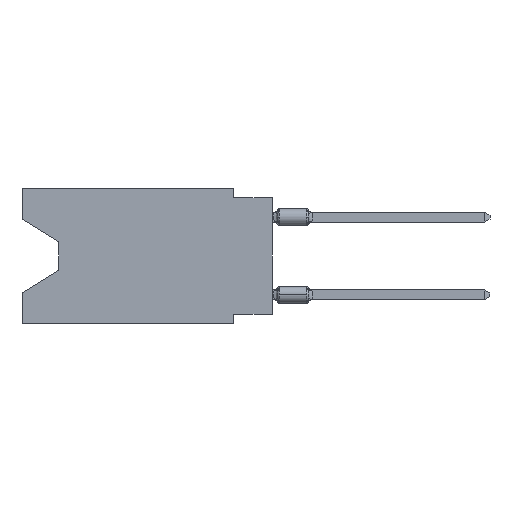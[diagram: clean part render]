
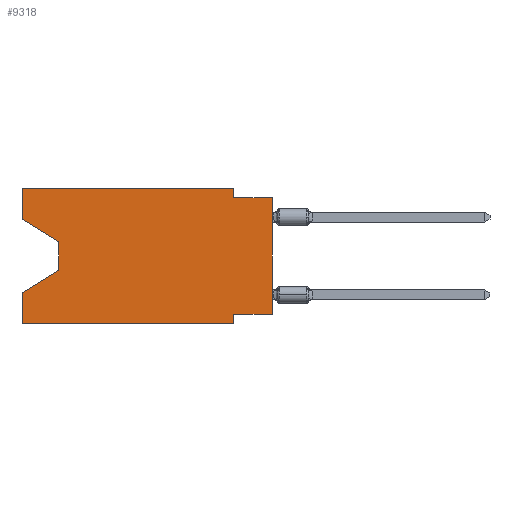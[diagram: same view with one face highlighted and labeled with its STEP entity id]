
A CAD part, left-side view. The second image highlights one B-rep face of the part: STEP entity #9318.
In plain terms, the highlighted planar face has unit normal (-1, 0, 0).
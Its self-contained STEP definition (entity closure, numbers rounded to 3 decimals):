
#119 = DIRECTION ( 'NONE',  ( 0., -0.855, -0.519 ) ) ;
#286 = CARTESIAN_POINT ( 'NONE',  ( 0., 16.383, 0. ) ) ;
#293 = VECTOR ( 'NONE', #8995, 1000. ) ;
#487 = EDGE_LOOP ( 'NONE', ( #8779, #12676, #13603, #1640, #14141, #2766, #3883, #6913, #11118, #13577, #760, #15820 ) ) ;
#689 = EDGE_CURVE ( 'NONE', #14110, #15507, #8025, .T. ) ;
#760 = ORIENTED_EDGE ( 'NONE', *, *, #9968, .F. ) ;
#988 = CARTESIAN_POINT ( 'NONE',  ( 0., 2.54, -8.89 ) ) ;
#1004 = VERTEX_POINT ( 'NONE', #4857 ) ;
#1427 = DIRECTION ( 'NONE',  ( 0., 0., -1. ) ) ;
#1616 = CARTESIAN_POINT ( 'NONE',  ( 0., 16.383, -8.89 ) ) ;
#1617 = AXIS2_PLACEMENT_3D ( 'NONE', #15998, #2168, #8337 ) ;
#1640 = ORIENTED_EDGE ( 'NONE', *, *, #5304, .F. ) ;
#1665 = LINE ( 'NONE', #4486, #16188 ) ;
#1762 = CARTESIAN_POINT ( 'NONE',  ( 0., 13.97, -5.385 ) ) ;
#1956 = VECTOR ( 'NONE', #12946, 1000. ) ;
#2101 = VECTOR ( 'NONE', #9533, 1000. ) ;
#2168 = DIRECTION ( 'NONE',  ( 1., 0., 0. ) ) ;
#2461 = VERTEX_POINT ( 'NONE', #4972 ) ;
#2766 = ORIENTED_EDGE ( 'NONE', *, *, #3567, .F. ) ;
#2842 = CARTESIAN_POINT ( 'NONE',  ( 0., 16.383, 0. ) ) ;
#2948 = CARTESIAN_POINT ( 'NONE',  ( 0., 0., -0.635 ) ) ;
#3024 = EDGE_CURVE ( 'NONE', #15430, #4402, #8748, .T. ) ;
#3173 = EDGE_CURVE ( 'NONE', #15507, #14469, #10854, .T. ) ;
#3236 = CARTESIAN_POINT ( 'NONE',  ( 0., 2.54, 0. ) ) ;
#3567 = EDGE_CURVE ( 'NONE', #1004, #7500, #13640, .T. ) ;
#3883 = ORIENTED_EDGE ( 'NONE', *, *, #8010, .F. ) ;
#3884 = LINE ( 'NONE', #1616, #17358 ) ;
#3995 = EDGE_CURVE ( 'NONE', #13683, #7500, #3884, .T. ) ;
#4402 = VERTEX_POINT ( 'NONE', #15620 ) ;
#4486 = CARTESIAN_POINT ( 'NONE',  ( 0., 0., -8.255 ) ) ;
#4857 = CARTESIAN_POINT ( 'NONE',  ( 0., 2.54, -8.255 ) ) ;
#4900 = CARTESIAN_POINT ( 'NONE',  ( 0., 16.383, -6.852 ) ) ;
#4905 = DIRECTION ( 'NONE',  ( 0., 0.855, -0.519 ) ) ;
#4957 = EDGE_CURVE ( 'NONE', #2461, #18977, #6547, .T. ) ;
#4972 = CARTESIAN_POINT ( 'NONE',  ( 0., 16.383, -2.038 ) ) ;
#5265 = CARTESIAN_POINT ( 'NONE',  ( 0., 13.97, -3.505 ) ) ;
#5304 = EDGE_CURVE ( 'NONE', #13683, #14469, #6423, .T. ) ;
#5669 = CARTESIAN_POINT ( 'NONE',  ( 0., 16.383, -8.89 ) ) ;
#5997 = DIRECTION ( 'NONE',  ( 0., 0., -1. ) ) ;
#6281 = CARTESIAN_POINT ( 'NONE',  ( 0., 2.54, -8.89 ) ) ;
#6423 = LINE ( 'NONE', #11070, #12446 ) ;
#6497 = CARTESIAN_POINT ( 'NONE',  ( 0., 13.97, -3.505 ) ) ;
#6547 = LINE ( 'NONE', #286, #9567 ) ;
#6851 = CARTESIAN_POINT ( 'NONE',  ( 0., 13.97, -5.385 ) ) ;
#6913 = ORIENTED_EDGE ( 'NONE', *, *, #9634, .T. ) ;
#7500 = VERTEX_POINT ( 'NONE', #988 ) ;
#7670 = VECTOR ( 'NONE', #4905, 1000. ) ;
#8010 = EDGE_CURVE ( 'NONE', #14268, #1004, #1665, .T. ) ;
#8025 = LINE ( 'NONE', #6497, #2101 ) ;
#8315 = LINE ( 'NONE', #9526, #1956 ) ;
#8337 = DIRECTION ( 'NONE',  ( 0., 0., -1. ) ) ;
#8748 = LINE ( 'NONE', #13669, #19560 ) ;
#8779 = ORIENTED_EDGE ( 'NONE', *, *, #19073, .T. ) ;
#8995 = DIRECTION ( 'NONE',  ( 0., -1., 0. ) ) ;
#9318 = ADVANCED_FACE ( 'NONE', ( #11354 ), #9847, .F. ) ;
#9526 = CARTESIAN_POINT ( 'NONE',  ( 0., 0., 0. ) ) ;
#9533 = DIRECTION ( 'NONE',  ( 0., 0., -1. ) ) ;
#9567 = VECTOR ( 'NONE', #14119, 1000. ) ;
#9634 = EDGE_CURVE ( 'NONE', #14268, #19158, #8315, .T. ) ;
#9847 = PLANE ( 'NONE',  #1617 ) ;
#9968 = EDGE_CURVE ( 'NONE', #18977, #15430, #15447, .T. ) ;
#10450 = DIRECTION ( 'NONE',  ( 0., 1., 0. ) ) ;
#10854 = LINE ( 'NONE', #1762, #7670 ) ;
#10906 = DIRECTION ( 'NONE',  ( 0., -1., 0. ) ) ;
#11070 = CARTESIAN_POINT ( 'NONE',  ( 0., 16.383, 0. ) ) ;
#11118 = ORIENTED_EDGE ( 'NONE', *, *, #13830, .F. ) ;
#11354 = FACE_OUTER_BOUND ( 'NONE', #487, .T. ) ;
#12030 = CARTESIAN_POINT ( 'NONE',  ( 0., 16.383, -2.038 ) ) ;
#12446 = VECTOR ( 'NONE', #12779, 1000. ) ;
#12676 = ORIENTED_EDGE ( 'NONE', *, *, #689, .T. ) ;
#12779 = DIRECTION ( 'NONE',  ( 0., 0., 1. ) ) ;
#12826 = VECTOR ( 'NONE', #1427, 1000. ) ;
#12894 = VECTOR ( 'NONE', #119, 1000. ) ;
#12946 = DIRECTION ( 'NONE',  ( 0., 0., 1. ) ) ;
#13450 = CARTESIAN_POINT ( 'NONE',  ( 0., 16.383, 0. ) ) ;
#13577 = ORIENTED_EDGE ( 'NONE', *, *, #3024, .F. ) ;
#13603 = ORIENTED_EDGE ( 'NONE', *, *, #3173, .T. ) ;
#13640 = LINE ( 'NONE', #6281, #12826 ) ;
#13669 = CARTESIAN_POINT ( 'NONE',  ( 0., 2.54, 0. ) ) ;
#13683 = VERTEX_POINT ( 'NONE', #5669 ) ;
#13830 = EDGE_CURVE ( 'NONE', #4402, #19158, #16777, .T. ) ;
#13957 = LINE ( 'NONE', #12030, #12894 ) ;
#14110 = VERTEX_POINT ( 'NONE', #5265 ) ;
#14119 = DIRECTION ( 'NONE',  ( 0., 0., 1. ) ) ;
#14141 = ORIENTED_EDGE ( 'NONE', *, *, #3995, .T. ) ;
#14268 = VERTEX_POINT ( 'NONE', #16206 ) ;
#14469 = VERTEX_POINT ( 'NONE', #4900 ) ;
#15246 = DIRECTION ( 'NONE',  ( 0., -1., 0. ) ) ;
#15430 = VERTEX_POINT ( 'NONE', #3236 ) ;
#15447 = LINE ( 'NONE', #2842, #293 ) ;
#15507 = VERTEX_POINT ( 'NONE', #6851 ) ;
#15620 = CARTESIAN_POINT ( 'NONE',  ( 0., 2.54, -0.635 ) ) ;
#15820 = ORIENTED_EDGE ( 'NONE', *, *, #4957, .F. ) ;
#15998 = CARTESIAN_POINT ( 'NONE',  ( 0., 16.383, 0. ) ) ;
#16188 = VECTOR ( 'NONE', #10450, 1000. ) ;
#16206 = CARTESIAN_POINT ( 'NONE',  ( 0., 0., -8.255 ) ) ;
#16777 = LINE ( 'NONE', #2948, #18146 ) ;
#17287 = CARTESIAN_POINT ( 'NONE',  ( 0., 0., -0.635 ) ) ;
#17358 = VECTOR ( 'NONE', #10906, 1000. ) ;
#18146 = VECTOR ( 'NONE', #15246, 1000. ) ;
#18977 = VERTEX_POINT ( 'NONE', #13450 ) ;
#19073 = EDGE_CURVE ( 'NONE', #2461, #14110, #13957, .T. ) ;
#19158 = VERTEX_POINT ( 'NONE', #17287 ) ;
#19560 = VECTOR ( 'NONE', #5997, 1000. ) ;
